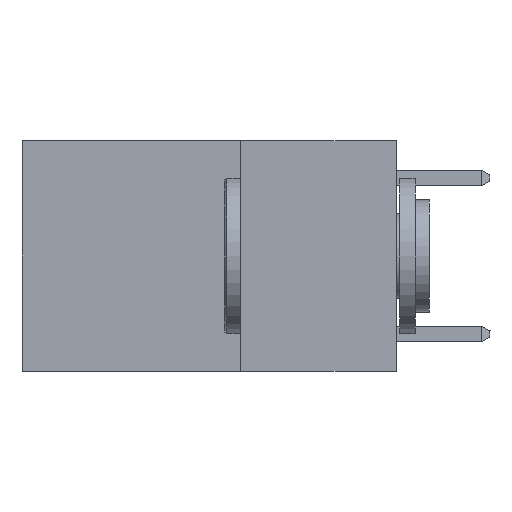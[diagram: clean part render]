
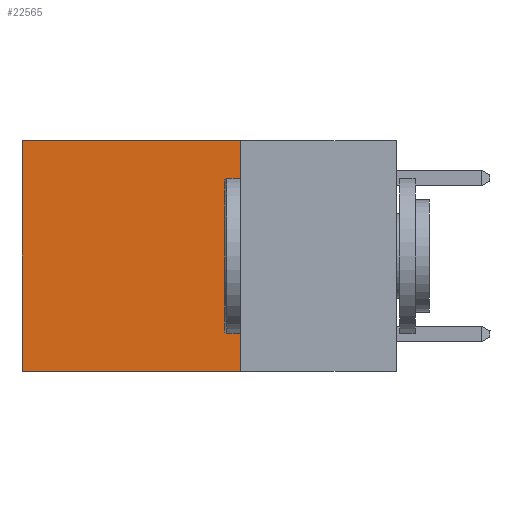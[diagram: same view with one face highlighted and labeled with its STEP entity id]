
A CAD part, left-side view. The second image highlights one B-rep face of the part: STEP entity #22565.
In plain terms, the highlighted planar face has unit normal (-1, 0, 0).
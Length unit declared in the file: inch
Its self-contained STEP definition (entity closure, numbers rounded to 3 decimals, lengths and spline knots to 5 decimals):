
#1080 = CARTESIAN_POINT ( 'NONE',  ( 0.2625, 0.25, -0.37 ) ) ;
#1098 = DIRECTION ( 'NONE',  ( 0., 0., -1. ) ) ;
#1438 = DIRECTION ( 'NONE',  ( 1., 0., 0. ) ) ;
#1955 = CARTESIAN_POINT ( 'NONE',  ( 0.2625, 0.6, -0.37 ) ) ;
#3766 = ORIENTED_EDGE ( 'NONE', *, *, #3829, .F. ) ;
#3818 = AXIS2_PLACEMENT_3D ( 'NONE', #27922, #1438, #17344 ) ;
#3829 = EDGE_CURVE ( 'NONE', #23698, #22727, #5690, .T. ) ;
#4662 = ORIENTED_EDGE ( 'NONE', *, *, #22051, .T. ) ;
#5690 = LINE ( 'NONE', #12788, #5722 ) ;
#5722 = VECTOR ( 'NONE', #8290, 39.37008 ) ;
#6287 = LINE ( 'NONE', #17758, #23235 ) ;
#8290 = DIRECTION ( 'NONE',  ( 0., 1., 0. ) ) ;
#8746 = LINE ( 'NONE', #13465, #20490 ) ;
#11588 = VERTEX_POINT ( 'NONE', #18621 ) ;
#12788 = CARTESIAN_POINT ( 'NONE',  ( 0.2625, 0.25, -0.37 ) ) ;
#12861 = PLANE ( 'NONE',  #3818 ) ;
#13465 = CARTESIAN_POINT ( 'NONE',  ( 0.2625, 0.25, 0. ) ) ;
#13620 = ORIENTED_EDGE ( 'NONE', *, *, #18107, .F. ) ;
#14119 = EDGE_LOOP ( 'NONE', ( #4662, #3766, #13620, #23444 ) ) ;
#15171 = VERTEX_POINT ( 'NONE', #20279 ) ;
#17344 = DIRECTION ( 'NONE',  ( 0., 0., -1. ) ) ;
#17758 = CARTESIAN_POINT ( 'NONE',  ( 0.2625, 0.6, 0. ) ) ;
#18107 = EDGE_CURVE ( 'NONE', #11588, #23698, #18986, .T. ) ;
#18621 = CARTESIAN_POINT ( 'NONE',  ( 0.2625, 0.25, 0. ) ) ;
#18986 = LINE ( 'NONE', #25569, #24042 ) ;
#20279 = CARTESIAN_POINT ( 'NONE',  ( 0.2625, 0.6, 0. ) ) ;
#20490 = VECTOR ( 'NONE', #26433, 39.37008 ) ;
#22051 = EDGE_CURVE ( 'NONE', #15171, #22727, #6287, .T. ) ;
#22565 = ADVANCED_FACE ( 'NONE', ( #27465 ), #12861, .F. ) ;
#22727 = VERTEX_POINT ( 'NONE', #1955 ) ;
#23235 = VECTOR ( 'NONE', #24157, 39.37008 ) ;
#23444 = ORIENTED_EDGE ( 'NONE', *, *, #28083, .T. ) ;
#23698 = VERTEX_POINT ( 'NONE', #1080 ) ;
#24042 = VECTOR ( 'NONE', #1098, 39.37008 ) ;
#24157 = DIRECTION ( 'NONE',  ( 0., 0., -1. ) ) ;
#25569 = CARTESIAN_POINT ( 'NONE',  ( 0.2625, 0.25, 0. ) ) ;
#26433 = DIRECTION ( 'NONE',  ( 0., 1., 0. ) ) ;
#27465 = FACE_OUTER_BOUND ( 'NONE', #14119, .T. ) ;
#27922 = CARTESIAN_POINT ( 'NONE',  ( 0.2625, 0.25, 0. ) ) ;
#28083 = EDGE_CURVE ( 'NONE', #11588, #15171, #8746, .T. ) ;
